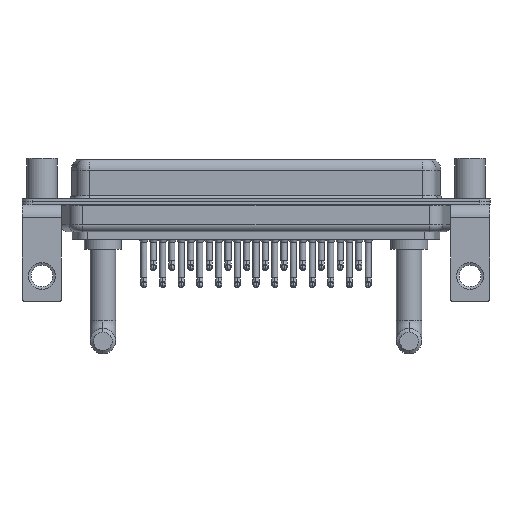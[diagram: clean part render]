
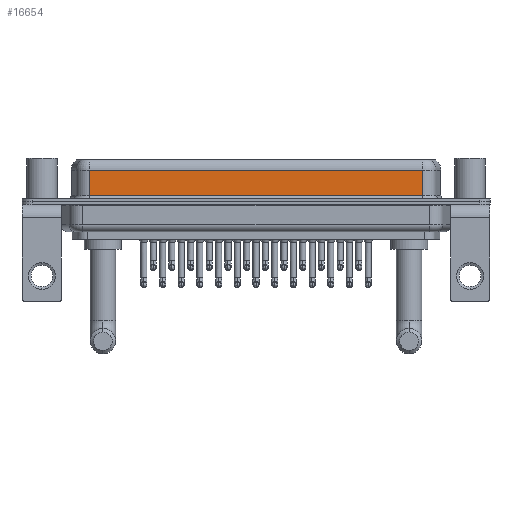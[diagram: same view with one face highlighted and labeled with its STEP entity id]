
A CAD part, front view. The second image highlights one B-rep face of the part: STEP entity #16654.
In plain terms, the highlighted planar face has unit normal (0, -1, 0).
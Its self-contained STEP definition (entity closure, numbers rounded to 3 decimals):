
#607 = VERTEX_POINT ( 'NONE', #24155 ) ;
#1148 = DIRECTION ( 'NONE',  ( 0., 0., 1. ) ) ;
#1480 = CARTESIAN_POINT ( 'NONE',  ( 56.462, -3.95, 0.9 ) ) ;
#3233 = PLANE ( 'NONE',  #13781 ) ;
#4434 = VECTOR ( 'NONE', #11568, 1000. ) ;
#4673 = EDGE_CURVE ( 'NONE', #607, #15221, #22205, .T. ) ;
#5209 = CARTESIAN_POINT ( 'NONE',  ( 56.462, -3.95, 4.65 ) ) ;
#5218 = CARTESIAN_POINT ( 'NONE',  ( 56.462, -3.95, 6.4 ) ) ;
#5292 = CARTESIAN_POINT ( 'NONE',  ( 7.038, -3.95, 6.4 ) ) ;
#5694 = CARTESIAN_POINT ( 'NONE',  ( 7.038, -3.95, 4.65 ) ) ;
#6943 = DIRECTION ( 'NONE',  ( 1., 0., 0. ) ) ;
#7635 = EDGE_CURVE ( 'NONE', #607, #19767, #24020, .T. ) ;
#10664 = CARTESIAN_POINT ( 'NONE',  ( 56.462, -3.95, 0.9 ) ) ;
#11568 = DIRECTION ( 'NONE',  ( 0., 0., -1. ) ) ;
#11640 = CARTESIAN_POINT ( 'NONE',  ( 56.462, -3.95, 6.4 ) ) ;
#12946 = VECTOR ( 'NONE', #21930, 1000. ) ;
#13338 = EDGE_LOOP ( 'NONE', ( #17012, #15591, #14272, #14962 ) ) ;
#13781 = AXIS2_PLACEMENT_3D ( 'NONE', #11640, #20082, #1148 ) ;
#14272 = ORIENTED_EDGE ( 'NONE', *, *, #25516, .T. ) ;
#14962 = ORIENTED_EDGE ( 'NONE', *, *, #15076, .T. ) ;
#15076 = EDGE_CURVE ( 'NONE', #19857, #19767, #20422, .T. ) ;
#15221 = VERTEX_POINT ( 'NONE', #5694 ) ;
#15359 = CARTESIAN_POINT ( 'NONE',  ( 7.038, -3.95, 0.9 ) ) ;
#15591 = ORIENTED_EDGE ( 'NONE', *, *, #4673, .T. ) ;
#16654 = ADVANCED_FACE ( 'NONE', ( #22156 ), #3233, .F. ) ;
#17012 = ORIENTED_EDGE ( 'NONE', *, *, #7635, .F. ) ;
#19767 = VERTEX_POINT ( 'NONE', #10664 ) ;
#19857 = VERTEX_POINT ( 'NONE', #15359 ) ;
#19879 = VECTOR ( 'NONE', #6943, 1000. ) ;
#19942 = DIRECTION ( 'NONE',  ( 0., 0., -1. ) ) ;
#20082 = DIRECTION ( 'NONE',  ( 0., 1., 0. ) ) ;
#20422 = LINE ( 'NONE', #1480, #19879 ) ;
#20482 = LINE ( 'NONE', #5292, #21525 ) ;
#21525 = VECTOR ( 'NONE', #19942, 1000. ) ;
#21930 = DIRECTION ( 'NONE',  ( -1., 0., 0. ) ) ;
#22156 = FACE_OUTER_BOUND ( 'NONE', #13338, .T. ) ;
#22205 = LINE ( 'NONE', #5209, #12946 ) ;
#24020 = LINE ( 'NONE', #5218, #4434 ) ;
#24155 = CARTESIAN_POINT ( 'NONE',  ( 56.462, -3.95, 4.65 ) ) ;
#25516 = EDGE_CURVE ( 'NONE', #15221, #19857, #20482, .T. ) ;
